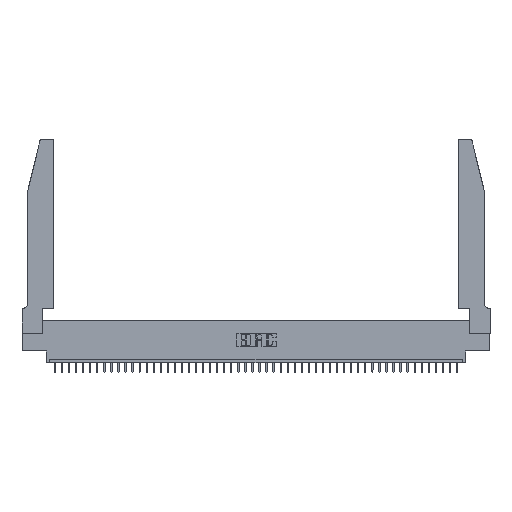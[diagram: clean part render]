
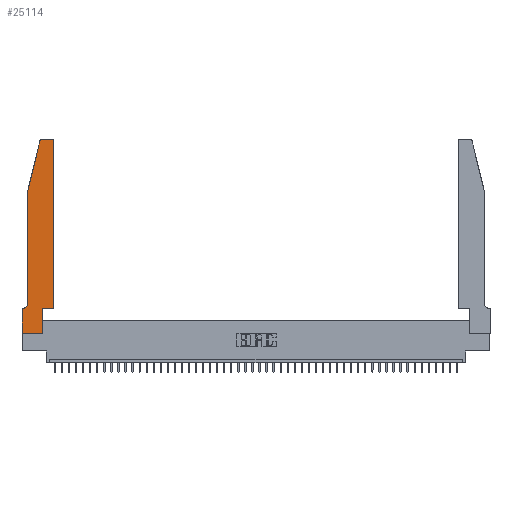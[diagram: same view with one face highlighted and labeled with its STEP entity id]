
A CAD part, top view. The second image highlights one B-rep face of the part: STEP entity #25114.
In plain terms, the highlighted planar face has unit normal (0, 0, 1).
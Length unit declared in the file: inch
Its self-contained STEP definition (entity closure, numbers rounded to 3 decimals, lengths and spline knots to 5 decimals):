
#1565 = DIRECTION ( 'NONE',  ( 0., 1., 0. ) ) ;
#1575 = CARTESIAN_POINT ( 'NONE',  ( 0., 0., 0.37 ) ) ;
#1829 = DIRECTION ( 'NONE',  ( 1., 0., 0. ) ) ;
#2117 = CARTESIAN_POINT ( 'NONE',  ( 0.4505, 0.35, 0.37 ) ) ;
#2272 = CARTESIAN_POINT ( 'NONE',  ( 0.2865, 0.35, 0.37 ) ) ;
#2717 = CARTESIAN_POINT ( 'NONE',  ( 0.0755, 0.35, 0.37 ) ) ;
#3064 = ORIENTED_EDGE ( 'NONE', *, *, #43114, .T. ) ;
#3146 = CARTESIAN_POINT ( 'NONE',  ( 0.284, 2.75, 0.37 ) ) ;
#3920 = CARTESIAN_POINT ( 'NONE',  ( 0.0755, 0.42, 0.37 ) ) ;
#4296 = EDGE_CURVE ( 'NONE', #16758, #15915, #12646, .T. ) ;
#4358 = ORIENTED_EDGE ( 'NONE', *, *, #23625, .T. ) ;
#6054 = DIRECTION ( 'NONE',  ( -1., 0., 0. ) ) ;
#10077 = ORIENTED_EDGE ( 'NONE', *, *, #44457, .T. ) ;
#10289 = CIRCLE ( 'NONE', #11756, 0.03 ) ;
#10521 = CARTESIAN_POINT ( 'NONE',  ( 0.0755, 2., 0.37 ) ) ;
#10903 = VECTOR ( 'NONE', #15907, 39.37008 ) ;
#11419 = CARTESIAN_POINT ( 'NONE',  ( 0.4505, 0.35, 0.37 ) ) ;
#11632 = ORIENTED_EDGE ( 'NONE', *, *, #17642, .T. ) ;
#11756 = AXIS2_PLACEMENT_3D ( 'NONE', #17773, #29033, #28794 ) ;
#12147 = LINE ( 'NONE', #1575, #10903 ) ;
#12324 = DIRECTION ( 'NONE',  ( 1., 0., 0. ) ) ;
#12646 = LINE ( 'NONE', #26773, #46319 ) ;
#12692 = ORIENTED_EDGE ( 'NONE', *, *, #12997, .T. ) ;
#12997 = EDGE_CURVE ( 'NONE', #23078, #32115, #16346, .T. ) ;
#13343 = VERTEX_POINT ( 'NONE', #40551 ) ;
#13386 = DIRECTION ( 'NONE',  ( 1., 0., 0. ) ) ;
#13527 = CARTESIAN_POINT ( 'NONE',  ( 0.0055, 0.35, 0.37 ) ) ;
#13910 = VECTOR ( 'NONE', #24292, 39.37008 ) ;
#13950 = LINE ( 'NONE', #21455, #13910 ) ;
#14023 = CARTESIAN_POINT ( 'NONE',  ( 0.2865, 0., 0.37 ) ) ;
#14168 = CARTESIAN_POINT ( 'NONE',  ( 0.2605, 2.75, 0.37 ) ) ;
#14359 = EDGE_CURVE ( 'NONE', #16774, #23078, #31622, .T. ) ;
#14829 = ORIENTED_EDGE ( 'NONE', *, *, #24430, .T. ) ;
#15249 = CARTESIAN_POINT ( 'NONE',  ( 0.4505, 2.72, 0.37 ) ) ;
#15862 = CARTESIAN_POINT ( 'NONE',  ( 0.4205, 2.72, 0.37 ) ) ;
#15907 = DIRECTION ( 'NONE',  ( 1., 0., 0. ) ) ;
#15915 = VERTEX_POINT ( 'NONE', #11419 ) ;
#16102 = VECTOR ( 'NONE', #1565, 39.37008 ) ;
#16346 = LINE ( 'NONE', #45502, #43987 ) ;
#16374 = CIRCLE ( 'NONE', #41904, 0.07 ) ;
#16524 = CARTESIAN_POINT ( 'NONE',  ( 0., 0., 0.37 ) ) ;
#16758 = VERTEX_POINT ( 'NONE', #46208 ) ;
#16774 = VERTEX_POINT ( 'NONE', #13527 ) ;
#16912 = FACE_OUTER_BOUND ( 'NONE', #42771, .T. ) ;
#17220 = ORIENTED_EDGE ( 'NONE', *, *, #4296, .T. ) ;
#17642 = EDGE_CURVE ( 'NONE', #24874, #19904, #46280, .T. ) ;
#17744 = AXIS2_PLACEMENT_3D ( 'NONE', #31253, #45601, #13386 ) ;
#17773 = CARTESIAN_POINT ( 'NONE',  ( 0.284, 2.72, 0.37 ) ) ;
#18133 = ORIENTED_EDGE ( 'NONE', *, *, #38377, .T. ) ;
#18519 = EDGE_CURVE ( 'NONE', #19904, #36994, #13950, .T. ) ;
#19432 = LINE ( 'NONE', #2272, #16102 ) ;
#19729 = PLANE ( 'NONE',  #17744 ) ;
#19904 = VERTEX_POINT ( 'NONE', #22390 ) ;
#21048 = EDGE_CURVE ( 'NONE', #15915, #37876, #24207, .T. ) ;
#21455 = CARTESIAN_POINT ( 'NONE',  ( 0.0755, 2., 0.37 ) ) ;
#22390 = CARTESIAN_POINT ( 'NONE',  ( 0.0755, 2., 0.37 ) ) ;
#23078 = VERTEX_POINT ( 'NONE', #45275 ) ;
#23625 = EDGE_CURVE ( 'NONE', #13343, #42320, #30863, .T. ) ;
#24207 = LINE ( 'NONE', #2117, #27348 ) ;
#24292 = DIRECTION ( 'NONE',  ( 0., -1., 0. ) ) ;
#24430 = EDGE_CURVE ( 'NONE', #32115, #31449, #12147, .T. ) ;
#24570 = DIRECTION ( 'NONE',  ( 0., -1., 0. ) ) ;
#24874 = VERTEX_POINT ( 'NONE', #36013 ) ;
#25114 = ADVANCED_FACE ( 'NONE', ( #16912 ), #19729, .T. ) ;
#26773 = CARTESIAN_POINT ( 'NONE',  ( 0.4505, 0.35, 0.37 ) ) ;
#27348 = VECTOR ( 'NONE', #34571, 39.37008 ) ;
#27903 = DIRECTION ( 'NONE',  ( 0., 0., -1. ) ) ;
#28794 = DIRECTION ( 'NONE',  ( 1., 0., 0. ) ) ;
#29033 = DIRECTION ( 'NONE',  ( 0., 0., 1. ) ) ;
#30863 = LINE ( 'NONE', #14168, #38682 ) ;
#31253 = CARTESIAN_POINT ( 'NONE',  ( 0., 0.35, 0.37 ) ) ;
#31449 = VERTEX_POINT ( 'NONE', #14023 ) ;
#31622 = LINE ( 'NONE', #2717, #35868 ) ;
#32115 = VERTEX_POINT ( 'NONE', #16524 ) ;
#32927 = ORIENTED_EDGE ( 'NONE', *, *, #44765, .T. ) ;
#34571 = DIRECTION ( 'NONE',  ( 0., 1., 0. ) ) ;
#35868 = VECTOR ( 'NONE', #45964, 39.37008 ) ;
#35930 = AXIS2_PLACEMENT_3D ( 'NONE', #15862, #44557, #12324 ) ;
#36013 = CARTESIAN_POINT ( 'NONE',  ( 0.25487, 2.72718, 0.37 ) ) ;
#36994 = VERTEX_POINT ( 'NONE', #3920 ) ;
#37876 = VERTEX_POINT ( 'NONE', #15249 ) ;
#38377 = EDGE_CURVE ( 'NONE', #31449, #16758, #19432, .T. ) ;
#38667 = VECTOR ( 'NONE', #39241, 39.37008 ) ;
#38682 = VECTOR ( 'NONE', #39115, 39.37008 ) ;
#39115 = DIRECTION ( 'NONE',  ( -1., 0., 0. ) ) ;
#39241 = DIRECTION ( 'NONE',  ( -0.239, -0.971, 0. ) ) ;
#39713 = ORIENTED_EDGE ( 'NONE', *, *, #21048, .T. ) ;
#40551 = CARTESIAN_POINT ( 'NONE',  ( 0.4205, 2.75, 0.37 ) ) ;
#41904 = AXIS2_PLACEMENT_3D ( 'NONE', #45322, #27903, #6054 ) ;
#41981 = ORIENTED_EDGE ( 'NONE', *, *, #18519, .T. ) ;
#42320 = VERTEX_POINT ( 'NONE', #3146 ) ;
#42771 = EDGE_LOOP ( 'NONE', ( #4358, #3064, #11632, #41981, #10077, #45534, #12692, #14829, #18133, #17220, #39713, #32927 ) ) ;
#43114 = EDGE_CURVE ( 'NONE', #42320, #24874, #10289, .T. ) ;
#43987 = VECTOR ( 'NONE', #24570, 39.37008 ) ;
#44457 = EDGE_CURVE ( 'NONE', #36994, #16774, #16374, .T. ) ;
#44557 = DIRECTION ( 'NONE',  ( 0., 0., 1. ) ) ;
#44765 = EDGE_CURVE ( 'NONE', #37876, #13343, #45684, .T. ) ;
#45275 = CARTESIAN_POINT ( 'NONE',  ( 0., 0.35, 0.37 ) ) ;
#45322 = CARTESIAN_POINT ( 'NONE',  ( 0.0055, 0.42, 0.37 ) ) ;
#45502 = CARTESIAN_POINT ( 'NONE',  ( 0., 0., 0.37 ) ) ;
#45534 = ORIENTED_EDGE ( 'NONE', *, *, #14359, .T. ) ;
#45601 = DIRECTION ( 'NONE',  ( 0., 0., 1. ) ) ;
#45684 = CIRCLE ( 'NONE', #35930, 0.03 ) ;
#45964 = DIRECTION ( 'NONE',  ( -1., 0., 0. ) ) ;
#46208 = CARTESIAN_POINT ( 'NONE',  ( 0.2865, 0.35, 0.37 ) ) ;
#46280 = LINE ( 'NONE', #10521, #38667 ) ;
#46319 = VECTOR ( 'NONE', #1829, 39.37008 ) ;
